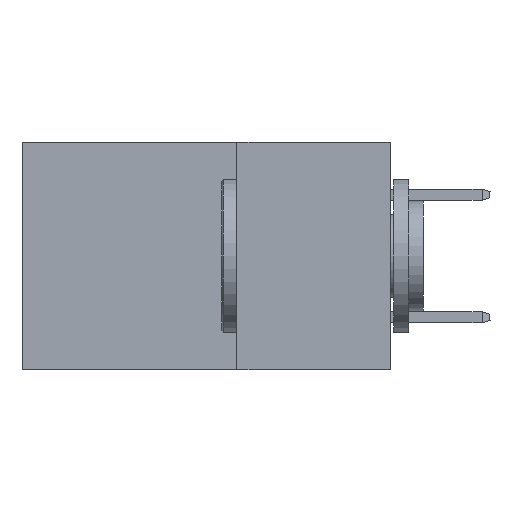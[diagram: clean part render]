
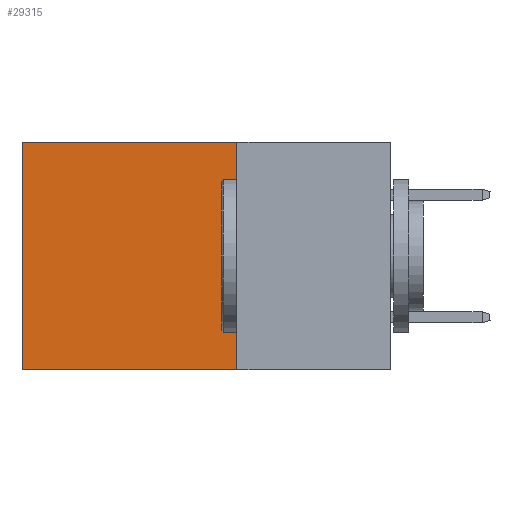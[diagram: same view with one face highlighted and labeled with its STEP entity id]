
A CAD part, left-side view. The second image highlights one B-rep face of the part: STEP entity #29315.
In plain terms, the highlighted planar face has unit normal (-1, 0, 0).
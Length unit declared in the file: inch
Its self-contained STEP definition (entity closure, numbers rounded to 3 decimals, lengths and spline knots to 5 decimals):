
#609 = VERTEX_POINT ( 'NONE', #39142 ) ;
#859 = FACE_OUTER_BOUND ( 'NONE', #31045, .T. ) ;
#7892 = VERTEX_POINT ( 'NONE', #28430 ) ;
#8446 = DIRECTION ( 'NONE',  ( 0., 0., -1. ) ) ;
#8470 = VERTEX_POINT ( 'NONE', #24869 ) ;
#12355 = CARTESIAN_POINT ( 'NONE',  ( 0.2875, 0.6, 0. ) ) ;
#12759 = LINE ( 'NONE', #35205, #29709 ) ;
#13183 = EDGE_CURVE ( 'NONE', #32567, #609, #12759, .T. ) ;
#15016 = CARTESIAN_POINT ( 'NONE',  ( 0.2875, 0.25, 0. ) ) ;
#17066 = DIRECTION ( 'NONE',  ( 0., 0., -1. ) ) ;
#20818 = DIRECTION ( 'NONE',  ( 0., 1., 0. ) ) ;
#22401 = EDGE_CURVE ( 'NONE', #7892, #32567, #24875, .T. ) ;
#23179 = DIRECTION ( 'NONE',  ( 0., 0., -1. ) ) ;
#23416 = ORIENTED_EDGE ( 'NONE', *, *, #39164, .T. ) ;
#23421 = LINE ( 'NONE', #15016, #24510 ) ;
#23945 = AXIS2_PLACEMENT_3D ( 'NONE', #34319, #34474, #17066 ) ;
#24147 = ORIENTED_EDGE ( 'NONE', *, *, #13183, .F. ) ;
#24510 = VECTOR ( 'NONE', #36205, 39.37008 ) ;
#24869 = CARTESIAN_POINT ( 'NONE',  ( 0.2875, 0.6, 0. ) ) ;
#24875 = LINE ( 'NONE', #43601, #29723 ) ;
#28430 = CARTESIAN_POINT ( 'NONE',  ( 0.2875, 0.25, 0. ) ) ;
#29315 = ADVANCED_FACE ( 'NONE', ( #859 ), #41434, .F. ) ;
#29709 = VECTOR ( 'NONE', #20818, 39.37008 ) ;
#29723 = VECTOR ( 'NONE', #23179, 39.37008 ) ;
#29738 = EDGE_CURVE ( 'NONE', #8470, #609, #44080, .T. ) ;
#31045 = EDGE_LOOP ( 'NONE', ( #34324, #24147, #37151, #23416 ) ) ;
#32567 = VERTEX_POINT ( 'NONE', #41958 ) ;
#34319 = CARTESIAN_POINT ( 'NONE',  ( 0.2875, 0.25, 0. ) ) ;
#34324 = ORIENTED_EDGE ( 'NONE', *, *, #29738, .T. ) ;
#34474 = DIRECTION ( 'NONE',  ( 1., 0., 0. ) ) ;
#34887 = VECTOR ( 'NONE', #8446, 39.37008 ) ;
#35205 = CARTESIAN_POINT ( 'NONE',  ( 0.2875, 0.25, -0.37 ) ) ;
#36205 = DIRECTION ( 'NONE',  ( 0., 1., 0. ) ) ;
#37151 = ORIENTED_EDGE ( 'NONE', *, *, #22401, .F. ) ;
#39142 = CARTESIAN_POINT ( 'NONE',  ( 0.2875, 0.6, -0.37 ) ) ;
#39164 = EDGE_CURVE ( 'NONE', #7892, #8470, #23421, .T. ) ;
#41434 = PLANE ( 'NONE',  #23945 ) ;
#41958 = CARTESIAN_POINT ( 'NONE',  ( 0.2875, 0.25, -0.37 ) ) ;
#43601 = CARTESIAN_POINT ( 'NONE',  ( 0.2875, 0.25, 0. ) ) ;
#44080 = LINE ( 'NONE', #12355, #34887 ) ;
